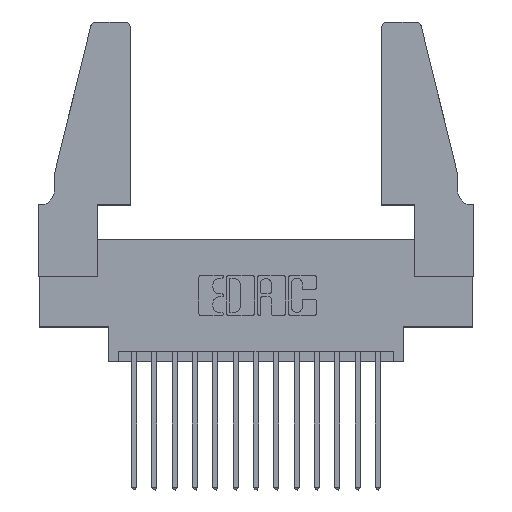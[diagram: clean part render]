
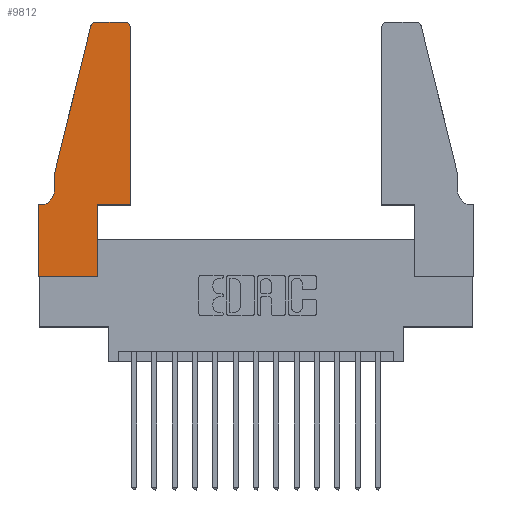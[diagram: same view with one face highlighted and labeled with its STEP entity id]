
A CAD part, top view. The second image highlights one B-rep face of the part: STEP entity #9812.
In plain terms, the highlighted planar face has unit normal (0, 0, 1).
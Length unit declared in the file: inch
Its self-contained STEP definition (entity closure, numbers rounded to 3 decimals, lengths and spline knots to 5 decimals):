
#512 = DIRECTION ( 'NONE',  ( 0., 0., 1. ) ) ;
#621 = VECTOR ( 'NONE', #11756, 39.37008 ) ;
#647 = CARTESIAN_POINT ( 'NONE',  ( 0.0755, 0.5, 0.37 ) ) ;
#699 = DIRECTION ( 'NONE',  ( 0., 0., 1. ) ) ;
#794 = CARTESIAN_POINT ( 'NONE',  ( 0.0755, 0.5, 0.37 ) ) ;
#891 = VECTOR ( 'NONE', #8418, 39.37008 ) ;
#947 = VERTEX_POINT ( 'NONE', #2304 ) ;
#1062 = EDGE_CURVE ( 'NONE', #8034, #6079, #1749, .T. ) ;
#1313 = EDGE_CURVE ( 'NONE', #2630, #15757, #4956, .T. ) ;
#1581 = VERTEX_POINT ( 'NONE', #12709 ) ;
#1610 = CARTESIAN_POINT ( 'NONE',  ( 0.2865, 0.35, 0.37 ) ) ;
#1670 = CIRCLE ( 'NONE', #2184, 0.03 ) ;
#1749 = CIRCLE ( 'NONE', #5049, 0.03 ) ;
#1795 = LINE ( 'NONE', #4550, #14903 ) ;
#1849 = VECTOR ( 'NONE', #14894, 39.37008 ) ;
#1877 = CARTESIAN_POINT ( 'NONE',  ( 0.2605, 1.25, 0.37 ) ) ;
#2077 = DIRECTION ( 'NONE',  ( 0., -1., 0. ) ) ;
#2184 = AXIS2_PLACEMENT_3D ( 'NONE', #8136, #512, #9412 ) ;
#2243 = CIRCLE ( 'NONE', #2875, 0.07 ) ;
#2266 = VERTEX_POINT ( 'NONE', #14222 ) ;
#2304 = CARTESIAN_POINT ( 'NONE',  ( 0., 0.35, 0.37 ) ) ;
#2630 = VERTEX_POINT ( 'NONE', #16227 ) ;
#2771 = VERTEX_POINT ( 'NONE', #8849 ) ;
#2811 = AXIS2_PLACEMENT_3D ( 'NONE', #3268, #699, #9600 ) ;
#2875 = AXIS2_PLACEMENT_3D ( 'NONE', #2988, #11807, #4278 ) ;
#2988 = CARTESIAN_POINT ( 'NONE',  ( 0.0055, 0.42, 0.37 ) ) ;
#3096 = EDGE_CURVE ( 'NONE', #15558, #9799, #11022, .T. ) ;
#3183 = DIRECTION ( 'NONE',  ( 0., 0., 1. ) ) ;
#3268 = CARTESIAN_POINT ( 'NONE',  ( 0., 0.35, 0.37 ) ) ;
#3625 = ORIENTED_EDGE ( 'NONE', *, *, #6629, .T. ) ;
#3696 = VECTOR ( 'NONE', #5723, 39.37008 ) ;
#3988 = VECTOR ( 'NONE', #8240, 39.37008 ) ;
#4205 = ORIENTED_EDGE ( 'NONE', *, *, #13012, .T. ) ;
#4278 = DIRECTION ( 'NONE',  ( -1., 0., 0. ) ) ;
#4345 = CARTESIAN_POINT ( 'NONE',  ( 0., 0., 0.37 ) ) ;
#4469 = LINE ( 'NONE', #1610, #621 ) ;
#4478 = CARTESIAN_POINT ( 'NONE',  ( 0.284, 1.25, 0.37 ) ) ;
#4550 = CARTESIAN_POINT ( 'NONE',  ( 0.0755, 0.5, 0.37 ) ) ;
#4588 = LINE ( 'NONE', #8393, #13883 ) ;
#4956 = LINE ( 'NONE', #4345, #3988 ) ;
#5049 = AXIS2_PLACEMENT_3D ( 'NONE', #10565, #3183, #13033 ) ;
#5723 = DIRECTION ( 'NONE',  ( -1., 0., 0. ) ) ;
#5837 = VERTEX_POINT ( 'NONE', #4478 ) ;
#5843 = EDGE_CURVE ( 'NONE', #6079, #5837, #7435, .T. ) ;
#6079 = VERTEX_POINT ( 'NONE', #13758 ) ;
#6467 = DIRECTION ( 'NONE',  ( 1., 0., 0. ) ) ;
#6629 = EDGE_CURVE ( 'NONE', #2266, #8034, #14945, .T. ) ;
#6681 = CARTESIAN_POINT ( 'NONE',  ( 0.2865, 0.35, 0.37 ) ) ;
#7039 = EDGE_CURVE ( 'NONE', #2771, #1581, #2243, .T. ) ;
#7378 = ORIENTED_EDGE ( 'NONE', *, *, #7793, .T. ) ;
#7435 = LINE ( 'NONE', #1877, #3696 ) ;
#7562 = VECTOR ( 'NONE', #13368, 39.37008 ) ;
#7793 = EDGE_CURVE ( 'NONE', #1581, #947, #10935, .T. ) ;
#8027 = ORIENTED_EDGE ( 'NONE', *, *, #14195, .T. ) ;
#8034 = VERTEX_POINT ( 'NONE', #12530 ) ;
#8136 = CARTESIAN_POINT ( 'NONE',  ( 0.284, 1.22, 0.37 ) ) ;
#8223 = ORIENTED_EDGE ( 'NONE', *, *, #9193, .T. ) ;
#8240 = DIRECTION ( 'NONE',  ( 1., 0., 0. ) ) ;
#8292 = ORIENTED_EDGE ( 'NONE', *, *, #8844, .T. ) ;
#8324 = PLANE ( 'NONE',  #2811 ) ;
#8393 = CARTESIAN_POINT ( 'NONE',  ( 0., 0., 0.37 ) ) ;
#8418 = DIRECTION ( 'NONE',  ( -0.239, -0.971, 0. ) ) ;
#8844 = EDGE_CURVE ( 'NONE', #11546, #2266, #16030, .T. ) ;
#8849 = CARTESIAN_POINT ( 'NONE',  ( 0.0755, 0.42, 0.37 ) ) ;
#8863 = FACE_OUTER_BOUND ( 'NONE', #10168, .T. ) ;
#9193 = EDGE_CURVE ( 'NONE', #947, #2630, #4588, .T. ) ;
#9287 = ORIENTED_EDGE ( 'NONE', *, *, #1313, .T. ) ;
#9412 = DIRECTION ( 'NONE',  ( 1., 0., 0. ) ) ;
#9600 = DIRECTION ( 'NONE',  ( 1., 0., 0. ) ) ;
#9696 = ORIENTED_EDGE ( 'NONE', *, *, #5843, .T. ) ;
#9724 = CARTESIAN_POINT ( 'NONE',  ( 0.2865, 0., 0.37 ) ) ;
#9768 = ORIENTED_EDGE ( 'NONE', *, *, #3096, .T. ) ;
#9799 = VERTEX_POINT ( 'NONE', #647 ) ;
#9812 = ADVANCED_FACE ( 'NONE', ( #8863 ), #8324, .T. ) ;
#10168 = EDGE_LOOP ( 'NONE', ( #9696, #4205, #9768, #11526, #12227, #7378, #8223, #9287, #8027, #8292, #3625, #14254 ) ) ;
#10565 = CARTESIAN_POINT ( 'NONE',  ( 0.4205, 1.22, 0.37 ) ) ;
#10797 = CARTESIAN_POINT ( 'NONE',  ( 0.0755, 0.35, 0.37 ) ) ;
#10825 = DIRECTION ( 'NONE',  ( 0., -1., 0. ) ) ;
#10935 = LINE ( 'NONE', #10797, #7562 ) ;
#11022 = LINE ( 'NONE', #794, #891 ) ;
#11526 = ORIENTED_EDGE ( 'NONE', *, *, #16225, .T. ) ;
#11546 = VERTEX_POINT ( 'NONE', #6681 ) ;
#11756 = DIRECTION ( 'NONE',  ( 0., 1., 0. ) ) ;
#11807 = DIRECTION ( 'NONE',  ( 0., 0., -1. ) ) ;
#12227 = ORIENTED_EDGE ( 'NONE', *, *, #7039, .T. ) ;
#12530 = CARTESIAN_POINT ( 'NONE',  ( 0.4505, 1.22, 0.37 ) ) ;
#12709 = CARTESIAN_POINT ( 'NONE',  ( 0.0055, 0.35, 0.37 ) ) ;
#12791 = CARTESIAN_POINT ( 'NONE',  ( 0.4505, 0.35, 0.37 ) ) ;
#13012 = EDGE_CURVE ( 'NONE', #5837, #15558, #1670, .T. ) ;
#13033 = DIRECTION ( 'NONE',  ( 1., 0., 0. ) ) ;
#13105 = VECTOR ( 'NONE', #6467, 39.37008 ) ;
#13368 = DIRECTION ( 'NONE',  ( -1., 0., 0. ) ) ;
#13628 = CARTESIAN_POINT ( 'NONE',  ( 0.4505, 0.35, 0.37 ) ) ;
#13758 = CARTESIAN_POINT ( 'NONE',  ( 0.4205, 1.25, 0.37 ) ) ;
#13883 = VECTOR ( 'NONE', #2077, 39.37008 ) ;
#14195 = EDGE_CURVE ( 'NONE', #15757, #11546, #4469, .T. ) ;
#14222 = CARTESIAN_POINT ( 'NONE',  ( 0.4505, 0.35, 0.37 ) ) ;
#14254 = ORIENTED_EDGE ( 'NONE', *, *, #1062, .T. ) ;
#14894 = DIRECTION ( 'NONE',  ( 0., 1., 0. ) ) ;
#14903 = VECTOR ( 'NONE', #10825, 39.37008 ) ;
#14945 = LINE ( 'NONE', #13628, #1849 ) ;
#15558 = VERTEX_POINT ( 'NONE', #15596 ) ;
#15596 = CARTESIAN_POINT ( 'NONE',  ( 0.25487, 1.22718, 0.37 ) ) ;
#15757 = VERTEX_POINT ( 'NONE', #9724 ) ;
#16030 = LINE ( 'NONE', #12791, #13105 ) ;
#16225 = EDGE_CURVE ( 'NONE', #9799, #2771, #1795, .T. ) ;
#16227 = CARTESIAN_POINT ( 'NONE',  ( 0., 0., 0.37 ) ) ;
